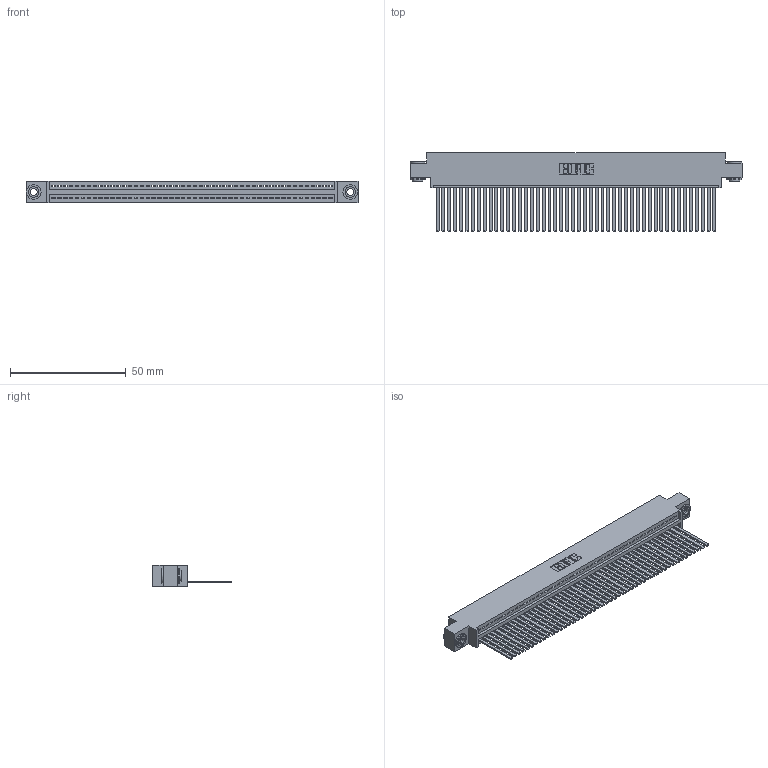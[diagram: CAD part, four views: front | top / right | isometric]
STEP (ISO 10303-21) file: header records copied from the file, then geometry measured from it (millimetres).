
FILE_DESCRIPTION (( 'STEP AP203' ), '1' );
FILE_NAME ('345-048-544-603.STEP', '2019-10-09T06:23:23', ( '' ), ( '' ), 'SwSTEP 2.0', 'SolidWorks 2016', '' );
FILE_SCHEMA (( 'CONFIG_CONTROL_DESIGN' ));
Length unit declared in the file: inch
Products named in the file (4): 345-048-544-603; 345-292-001_345-293-144; 345 Part_0.170 Offset - 0.156 Dia-TH; 345-250-002_345-250-002-102
Assembly tree (51 placements, depth 2):
  345-048-544-603
    345 Part_0.170 Offset - 0.156 Dia-TH
    345-292-001_345-293-144  x48
    345-250-002_345-250-002-102  x2
Bounding box: 143.13 x 33.96 x 9.4 mm (x, y, z)
Volume: 14105.6 mm3; surface area: 20836.5 mm2
Topology: 51 solids, 51 shells, 2664 faces, 8013 edges, 5274 vertices
Faces by surface type: plane 1822, cylinder 834, cone 8
Entity records: 35916 total; most frequent: CARTESIAN_POINT 6199, ORIENTED_EDGE 6174, DIRECTION 5433, EDGE_CURVE 3087, LINE 2743, VECTOR 2743, VERTEX_POINT 2054, AXIS2_PLACEMENT_3D 1345
